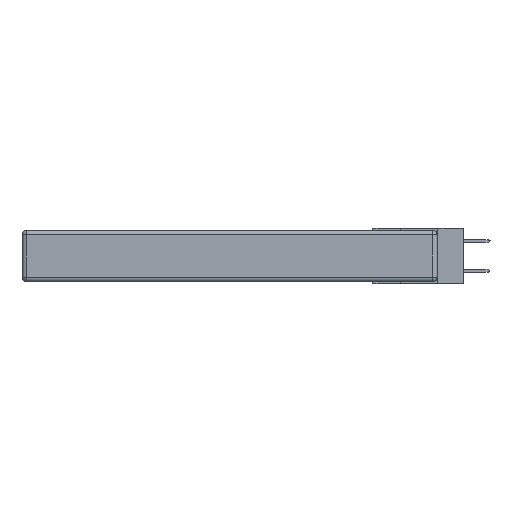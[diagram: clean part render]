
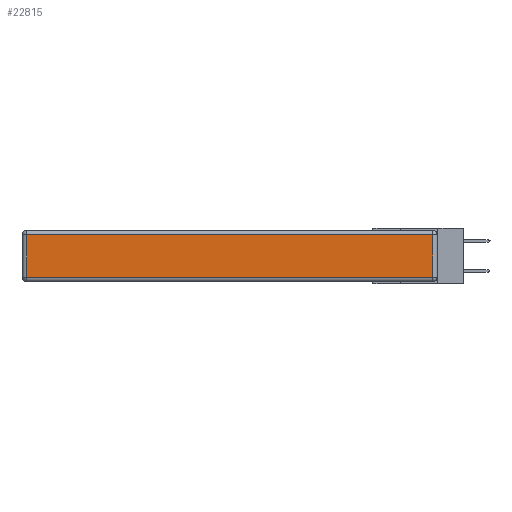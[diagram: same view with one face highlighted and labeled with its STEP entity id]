
A CAD part, left-side view. The second image highlights one B-rep face of the part: STEP entity #22815.
In plain terms, the highlighted planar face has unit normal (-1, 0, 0).
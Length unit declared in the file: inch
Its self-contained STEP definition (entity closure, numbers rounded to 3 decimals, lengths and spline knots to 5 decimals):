
#130 = CARTESIAN_POINT ( 'NONE',  ( 0., 2.72, -0.313 ) ) ;
#747 = LINE ( 'NONE', #13058, #22899 ) ;
#1055 = LINE ( 'NONE', #3082, #22855 ) ;
#1095 = EDGE_LOOP ( 'NONE', ( #21387, #25668, #22712, #20195 ) ) ;
#1809 = VECTOR ( 'NONE', #4897, 39.37008 ) ;
#2126 = CARTESIAN_POINT ( 'NONE',  ( 0., 2.75, -0.03 ) ) ;
#3082 = CARTESIAN_POINT ( 'NONE',  ( 0., 0.03, -0.343 ) ) ;
#3811 = VERTEX_POINT ( 'NONE', #8206 ) ;
#4897 = DIRECTION ( 'NONE',  ( 0., 0., -1. ) ) ;
#7308 = CARTESIAN_POINT ( 'NONE',  ( 0., 0., -0.343 ) ) ;
#8206 = CARTESIAN_POINT ( 'NONE',  ( 0., 0.03, -0.313 ) ) ;
#8579 = EDGE_CURVE ( 'NONE', #12367, #3811, #747, .T. ) ;
#9544 = DIRECTION ( 'NONE',  ( -1., 0., 0. ) ) ;
#11243 = VERTEX_POINT ( 'NONE', #18909 ) ;
#12367 = VERTEX_POINT ( 'NONE', #130 ) ;
#13058 = CARTESIAN_POINT ( 'NONE',  ( 0., 0., -0.313 ) ) ;
#14508 = VECTOR ( 'NONE', #20039, 39.37008 ) ;
#16137 = CARTESIAN_POINT ( 'NONE',  ( 0., 2.72, -0.343 ) ) ;
#16623 = EDGE_CURVE ( 'NONE', #11243, #12367, #19041, .T. ) ;
#18246 = FACE_OUTER_BOUND ( 'NONE', #1095, .T. ) ;
#18842 = DIRECTION ( 'NONE',  ( 0., 0., 1. ) ) ;
#18909 = CARTESIAN_POINT ( 'NONE',  ( 0., 2.72, -0.03 ) ) ;
#18979 = DIRECTION ( 'NONE',  ( 0., -1., 0. ) ) ;
#19041 = LINE ( 'NONE', #16137, #1809 ) ;
#20010 = EDGE_CURVE ( 'NONE', #3811, #25943, #1055, .T. ) ;
#20039 = DIRECTION ( 'NONE',  ( 0., 1., 0. ) ) ;
#20195 = ORIENTED_EDGE ( 'NONE', *, *, #16623, .T. ) ;
#20709 = PLANE ( 'NONE',  #25820 ) ;
#21387 = ORIENTED_EDGE ( 'NONE', *, *, #8579, .T. ) ;
#22712 = ORIENTED_EDGE ( 'NONE', *, *, #27576, .T. ) ;
#22815 = ADVANCED_FACE ( 'NONE', ( #18246 ), #20709, .T. ) ;
#22855 = VECTOR ( 'NONE', #18842, 39.37008 ) ;
#22899 = VECTOR ( 'NONE', #18979, 39.37008 ) ;
#25252 = DIRECTION ( 'NONE',  ( 0., 0., 1. ) ) ;
#25300 = CARTESIAN_POINT ( 'NONE',  ( 0., 0.03, -0.03 ) ) ;
#25383 = LINE ( 'NONE', #2126, #14508 ) ;
#25668 = ORIENTED_EDGE ( 'NONE', *, *, #20010, .T. ) ;
#25820 = AXIS2_PLACEMENT_3D ( 'NONE', #7308, #9544, #25252 ) ;
#25943 = VERTEX_POINT ( 'NONE', #25300 ) ;
#27576 = EDGE_CURVE ( 'NONE', #25943, #11243, #25383, .T. ) ;
